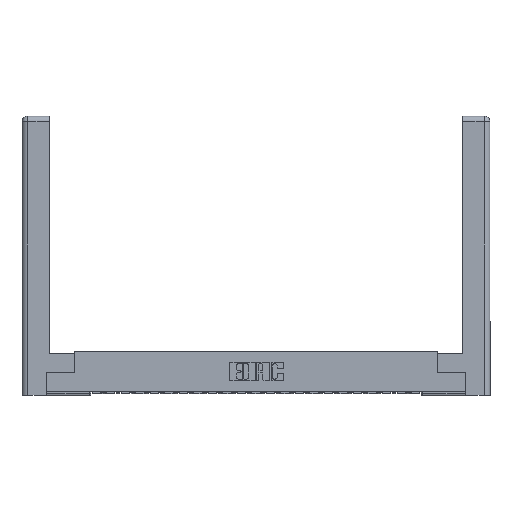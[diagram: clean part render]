
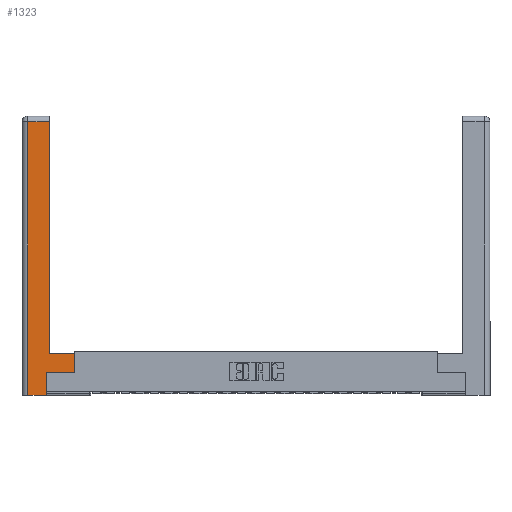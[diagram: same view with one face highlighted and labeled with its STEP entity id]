
A CAD part, top view. The second image highlights one B-rep face of the part: STEP entity #1323.
In plain terms, the highlighted planar face has unit normal (0, 0, 1).
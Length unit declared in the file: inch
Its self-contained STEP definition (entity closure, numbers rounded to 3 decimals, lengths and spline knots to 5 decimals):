
#217 = EDGE_CURVE ( 'NONE', #11658, #3507, #19739, .T. ) ;
#443 = ORIENTED_EDGE ( 'NONE', *, *, #13405, .T. ) ;
#656 = EDGE_CURVE ( 'NONE', #3507, #21250, #19082, .T. ) ;
#1323 = ADVANCED_FACE ( 'NONE', ( #16589 ), #8361, .F. ) ;
#1739 = ORIENTED_EDGE ( 'NONE', *, *, #22239, .T. ) ;
#1888 = CARTESIAN_POINT ( 'NONE',  ( 0.0615, 0., 0. ) ) ;
#2123 = DIRECTION ( 'NONE',  ( -1., 0., 0. ) ) ;
#2487 = CARTESIAN_POINT ( 'NONE',  ( 0.265, 0., 0. ) ) ;
#2490 = LINE ( 'NONE', #18539, #8990 ) ;
#2527 = DIRECTION ( 'NONE',  ( 1., 0., 0. ) ) ;
#2537 = VECTOR ( 'NONE', #25296, 39.37008 ) ;
#2940 = DIRECTION ( 'NONE',  ( 0., 1., 0. ) ) ;
#3259 = LINE ( 'NONE', #21838, #4783 ) ;
#3507 = VERTEX_POINT ( 'NONE', #3655 ) ;
#3593 = VECTOR ( 'NONE', #10563, 39.37008 ) ;
#3647 = VECTOR ( 'NONE', #5884, 39.37008 ) ;
#3655 = CARTESIAN_POINT ( 'NONE',  ( 0.0615, 2.94, 0. ) ) ;
#4121 = DIRECTION ( 'NONE',  ( 0., 0., -1. ) ) ;
#4587 = CARTESIAN_POINT ( 'NONE',  ( 0.0615, 0., 0. ) ) ;
#4783 = VECTOR ( 'NONE', #2123, 39.37008 ) ;
#4863 = DIRECTION ( 'NONE',  ( 0., 1., 0. ) ) ;
#5421 = VERTEX_POINT ( 'NONE', #11984 ) ;
#5688 = ORIENTED_EDGE ( 'NONE', *, *, #23738, .T. ) ;
#5884 = DIRECTION ( 'NONE',  ( -1., 0., 0. ) ) ;
#6352 = DIRECTION ( 'NONE',  ( -1., 0., 0. ) ) ;
#6760 = CARTESIAN_POINT ( 'NONE',  ( 0.565, 0.45, 0. ) ) ;
#8121 = VECTOR ( 'NONE', #19604, 39.37008 ) ;
#8361 = PLANE ( 'NONE',  #22388 ) ;
#8442 = CARTESIAN_POINT ( 'NONE',  ( 0.295, 0.45, 0. ) ) ;
#8990 = VECTOR ( 'NONE', #2527, 39.37008 ) ;
#9361 = CARTESIAN_POINT ( 'NONE',  ( 0.295, 3., 0. ) ) ;
#10010 = CARTESIAN_POINT ( 'NONE',  ( 0.295, 2.94, 0. ) ) ;
#10352 = CARTESIAN_POINT ( 'NONE',  ( 0.265, 0.245, 0. ) ) ;
#10563 = DIRECTION ( 'NONE',  ( 0., -1., 0. ) ) ;
#10829 = CARTESIAN_POINT ( 'NONE',  ( 0.265, 0.245, 0. ) ) ;
#11658 = VERTEX_POINT ( 'NONE', #10010 ) ;
#11984 = CARTESIAN_POINT ( 'NONE',  ( 0.565, 0.245, 0. ) ) ;
#11999 = ORIENTED_EDGE ( 'NONE', *, *, #19579, .T. ) ;
#12290 = LINE ( 'NONE', #6760, #13532 ) ;
#13297 = VECTOR ( 'NONE', #2940, 39.37008 ) ;
#13385 = LINE ( 'NONE', #19440, #8121 ) ;
#13405 = EDGE_CURVE ( 'NONE', #14296, #11658, #21428, .T. ) ;
#13532 = VECTOR ( 'NONE', #4863, 39.37008 ) ;
#14296 = VERTEX_POINT ( 'NONE', #8442 ) ;
#15145 = ORIENTED_EDGE ( 'NONE', *, *, #17326, .T. ) ;
#15997 = CARTESIAN_POINT ( 'NONE',  ( 0., 0., 0. ) ) ;
#16214 = CARTESIAN_POINT ( 'NONE',  ( 0.565, 0.45, 0. ) ) ;
#16589 = FACE_OUTER_BOUND ( 'NONE', #22904, .T. ) ;
#17261 = ORIENTED_EDGE ( 'NONE', *, *, #217, .T. ) ;
#17326 = EDGE_CURVE ( 'NONE', #21250, #24495, #13385, .T. ) ;
#17557 = ORIENTED_EDGE ( 'NONE', *, *, #18097, .T. ) ;
#18097 = EDGE_CURVE ( 'NONE', #20597, #5421, #2490, .T. ) ;
#18539 = CARTESIAN_POINT ( 'NONE',  ( 0.565, 0.245, 0. ) ) ;
#19082 = LINE ( 'NONE', #4587, #3593 ) ;
#19440 = CARTESIAN_POINT ( 'NONE',  ( 0.265, 0., 0. ) ) ;
#19449 = VERTEX_POINT ( 'NONE', #16214 ) ;
#19579 = EDGE_CURVE ( 'NONE', #24495, #20597, #19799, .T. ) ;
#19604 = DIRECTION ( 'NONE',  ( 1., 0., 0. ) ) ;
#19739 = LINE ( 'NONE', #21794, #3647 ) ;
#19799 = LINE ( 'NONE', #10829, #13297 ) ;
#20597 = VERTEX_POINT ( 'NONE', #10352 ) ;
#21250 = VERTEX_POINT ( 'NONE', #1888 ) ;
#21428 = LINE ( 'NONE', #9361, #2537 ) ;
#21794 = CARTESIAN_POINT ( 'NONE',  ( 0.0615, 2.94, 0. ) ) ;
#21838 = CARTESIAN_POINT ( 'NONE',  ( 0.295, 0.45, 0. ) ) ;
#22239 = EDGE_CURVE ( 'NONE', #5421, #19449, #12290, .T. ) ;
#22388 = AXIS2_PLACEMENT_3D ( 'NONE', #15997, #4121, #6352 ) ;
#22904 = EDGE_LOOP ( 'NONE', ( #443, #17261, #24556, #15145, #11999, #17557, #1739, #5688 ) ) ;
#23738 = EDGE_CURVE ( 'NONE', #19449, #14296, #3259, .T. ) ;
#24495 = VERTEX_POINT ( 'NONE', #2487 ) ;
#24556 = ORIENTED_EDGE ( 'NONE', *, *, #656, .T. ) ;
#25296 = DIRECTION ( 'NONE',  ( 0., 1., 0. ) ) ;
